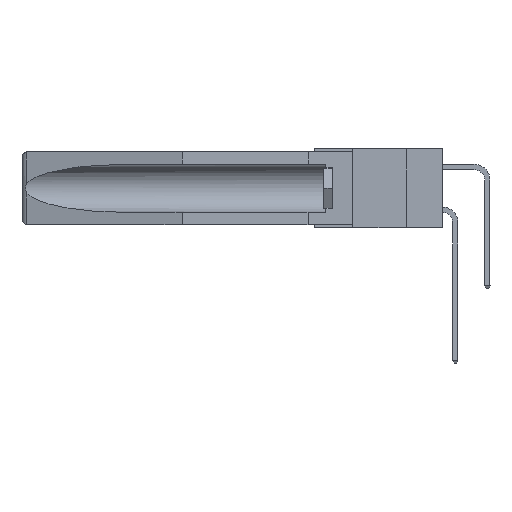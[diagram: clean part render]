
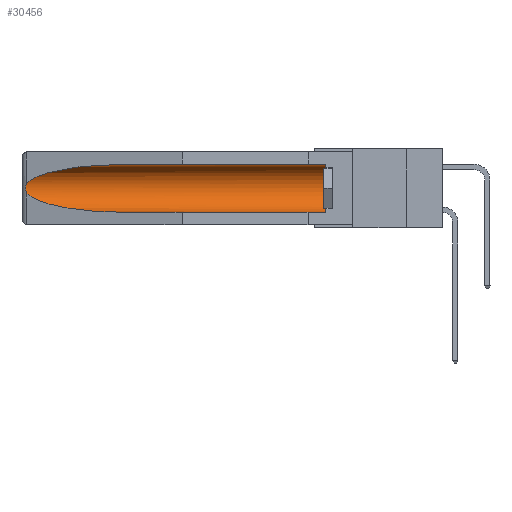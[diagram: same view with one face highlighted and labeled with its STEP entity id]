
A CAD part, left-side view. The second image highlights one B-rep face of the part: STEP entity #30456.
In plain terms, the highlighted cylindrical face has radius 2.857 mm (diameter 5.715 mm), a partial arc.
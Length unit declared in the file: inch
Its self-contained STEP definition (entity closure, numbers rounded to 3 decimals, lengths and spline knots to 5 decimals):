
#237 = CARTESIAN_POINT ( 'NONE',  ( 0.26537, 1.52718, -0.14972 ) ) ;
#562 = EDGE_LOOP ( 'NONE', ( #3902, #31738, #9379, #9687, #2522, #21869 ) ) ;
#686 = CARTESIAN_POINT ( 'NONE',  ( 0.25451, 1.48313, -0.09465 ) ) ;
#788 = VERTEX_POINT ( 'NONE', #17044 ) ;
#843 = DIRECTION ( 'NONE',  ( 0., 0., 1. ) ) ;
#1011 = CARTESIAN_POINT ( 'NONE',  ( 0.155, 1.07973, -0.059 ) ) ;
#1333 = VERTEX_POINT ( 'NONE', #5005 ) ;
#1341 = DIRECTION ( 'NONE',  ( 0., 0., 1. ) ) ;
#2293 =( BOUNDED_CURVE ( )  B_SPLINE_CURVE ( 3, ( #16032, #11132, #13650, #18616 ),
 .UNSPECIFIED., .F., .F. ) 
 B_SPLINE_CURVE_WITH_KNOTS ( ( 4, 4 ),
 ( 0.1948, 1.5708 ),
 .UNSPECIFIED. ) 
 CURVE ( )  GEOMETRIC_REPRESENTATION_ITEM ( )  RATIONAL_B_SPLINE_CURVE ( ( 1., 0.848, 0.848, 1. ) ) 
 REPRESENTATION_ITEM ( '' )  );
#2522 = ORIENTED_EDGE ( 'NONE', *, *, #29806, .T. ) ;
#3287 =( BOUNDED_CURVE ( )  B_SPLINE_CURVE ( 3, ( #5828, #5525, #686, #18017 ),
 .UNSPECIFIED., .F., .F. ) 
 B_SPLINE_CURVE_WITH_KNOTS ( ( 4, 4 ),
 ( 4.71239, 6.08839 ),
 .UNSPECIFIED. ) 
 CURVE ( )  GEOMETRIC_REPRESENTATION_ITEM ( )  RATIONAL_B_SPLINE_CURVE ( ( 1., 0.848, 0.848, 1. ) ) 
 REPRESENTATION_ITEM ( '' )  );
#3902 = ORIENTED_EDGE ( 'NONE', *, *, #16248, .T. ) ;
#4288 = LINE ( 'NONE', #28132, #20101 ) ;
#5005 = CARTESIAN_POINT ( 'NONE',  ( 0.155, 1.07973, -0.284 ) ) ;
#5525 = CARTESIAN_POINT ( 'NONE',  ( 0.21114, 1.30732, -0.059 ) ) ;
#5828 = CARTESIAN_POINT ( 'NONE',  ( 0.155, 1.07973, -0.059 ) ) ;
#6072 = DIRECTION ( 'NONE',  ( 0., 1., 0. ) ) ;
#7607 = CARTESIAN_POINT ( 'NONE',  ( 0.26654, 1.53092, -0.15636 ) ) ;
#8136 = CARTESIAN_POINT ( 'NONE',  ( 0.155, -0.30754, -0.284 ) ) ;
#8935 = VERTEX_POINT ( 'NONE', #25050 ) ;
#9158 = AXIS2_PLACEMENT_3D ( 'NONE', #30268, #10396, #843 ) ;
#9379 = ORIENTED_EDGE ( 'NONE', *, *, #16752, .T. ) ;
#9687 = ORIENTED_EDGE ( 'NONE', *, *, #20234, .F. ) ;
#10097 = CARTESIAN_POINT ( 'NONE',  ( 0.2673, 1.5327, -0.16383 ) ) ;
#10324 = CARTESIAN_POINT ( 'NONE',  ( 0.2675, 1.53308, -0.17534 ) ) ;
#10396 = DIRECTION ( 'NONE',  ( 0., 1., 0. ) ) ;
#11132 = CARTESIAN_POINT ( 'NONE',  ( 0.25451, 1.48313, -0.24835 ) ) ;
#12416 = CARTESIAN_POINT ( 'NONE',  ( 0.155, 0.126, -0.284 ) ) ;
#13650 = CARTESIAN_POINT ( 'NONE',  ( 0.21114, 1.30732, -0.284 ) ) ;
#14501 = CARTESIAN_POINT ( 'NONE',  ( 0.155, 0.126, -0.1715 ) ) ;
#15719 = EDGE_CURVE ( 'NONE', #8935, #23518, #16717, .T. ) ;
#15852 = VERTEX_POINT ( 'NONE', #1011 ) ;
#16032 = CARTESIAN_POINT ( 'NONE',  ( 0.26537, 1.52718, -0.19328 ) ) ;
#16095 = CYLINDRICAL_SURFACE ( 'NONE', #9158, 0.1125 ) ;
#16238 = VERTEX_POINT ( 'NONE', #12416 ) ;
#16248 = EDGE_CURVE ( 'NONE', #15852, #8935, #3287, .T. ) ;
#16717 = B_SPLINE_CURVE_WITH_KNOTS ( 'NONE', 3,
 ( #237, #22393, #7607, #10097, #25356, #10324, #29985, #20043, #30088, #20453 ),
 .UNSPECIFIED., .F., .F.,
 ( 4, 2, 2, 2, 4 ),
 ( 0., 0.00029, 0.00058, 0.00087, 0.00117 ),
 .UNSPECIFIED. ) ;
#16752 = EDGE_CURVE ( 'NONE', #23518, #1333, #2293, .T. ) ;
#16876 = LINE ( 'NONE', #8136, #19583 ) ;
#17044 = CARTESIAN_POINT ( 'NONE',  ( 0.155, 0.126, -0.059 ) ) ;
#18017 = CARTESIAN_POINT ( 'NONE',  ( 0.26537, 1.52718, -0.14972 ) ) ;
#18616 = CARTESIAN_POINT ( 'NONE',  ( 0.155, 1.07973, -0.284 ) ) ;
#18806 = DIRECTION ( 'NONE',  ( 0., -1., 0. ) ) ;
#19336 = CIRCLE ( 'NONE', #30182, 0.1125 ) ;
#19583 = VECTOR ( 'NONE', #25896, 39.37008 ) ;
#20043 = CARTESIAN_POINT ( 'NONE',  ( 0.26655, 1.53094, -0.18657 ) ) ;
#20101 = VECTOR ( 'NONE', #6072, 39.37008 ) ;
#20234 = EDGE_CURVE ( 'NONE', #16238, #1333, #16876, .T. ) ;
#20453 = CARTESIAN_POINT ( 'NONE',  ( 0.26537, 1.52718, -0.19328 ) ) ;
#21869 = ORIENTED_EDGE ( 'NONE', *, *, #29752, .T. ) ;
#22393 = CARTESIAN_POINT ( 'NONE',  ( 0.26597, 1.52961, -0.15275 ) ) ;
#23518 = VERTEX_POINT ( 'NONE', #27317 ) ;
#25050 = CARTESIAN_POINT ( 'NONE',  ( 0.26537, 1.52718, -0.14972 ) ) ;
#25356 = CARTESIAN_POINT ( 'NONE',  ( 0.2675, 1.53308, -0.16763 ) ) ;
#25896 = DIRECTION ( 'NONE',  ( 0., 1., 0. ) ) ;
#27317 = CARTESIAN_POINT ( 'NONE',  ( 0.26537, 1.52718, -0.19328 ) ) ;
#28132 = CARTESIAN_POINT ( 'NONE',  ( 0.155, -0.30754, -0.059 ) ) ;
#29138 = FACE_OUTER_BOUND ( 'NONE', #562, .T. ) ;
#29752 = EDGE_CURVE ( 'NONE', #788, #15852, #4288, .T. ) ;
#29806 = EDGE_CURVE ( 'NONE', #16238, #788, #19336, .T. ) ;
#29985 = CARTESIAN_POINT ( 'NONE',  ( 0.2673, 1.53269, -0.17917 ) ) ;
#30088 = CARTESIAN_POINT ( 'NONE',  ( 0.26597, 1.5296, -0.19026 ) ) ;
#30182 = AXIS2_PLACEMENT_3D ( 'NONE', #14501, #18806, #1341 ) ;
#30268 = CARTESIAN_POINT ( 'NONE',  ( 0.155, -0.30754, -0.1715 ) ) ;
#30456 = ADVANCED_FACE ( 'NONE', ( #29138 ), #16095, .F. ) ;
#31738 = ORIENTED_EDGE ( 'NONE', *, *, #15719, .T. ) ;
